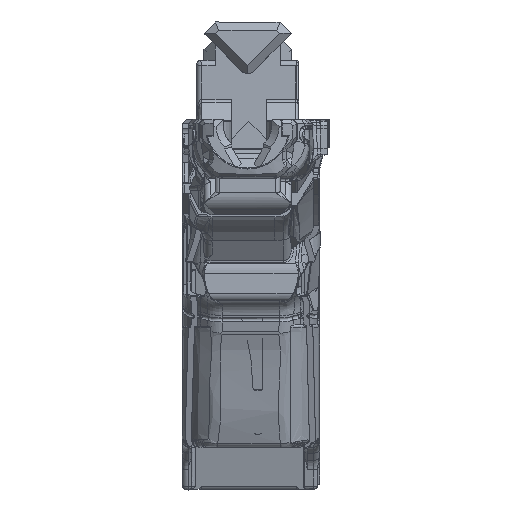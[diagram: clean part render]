
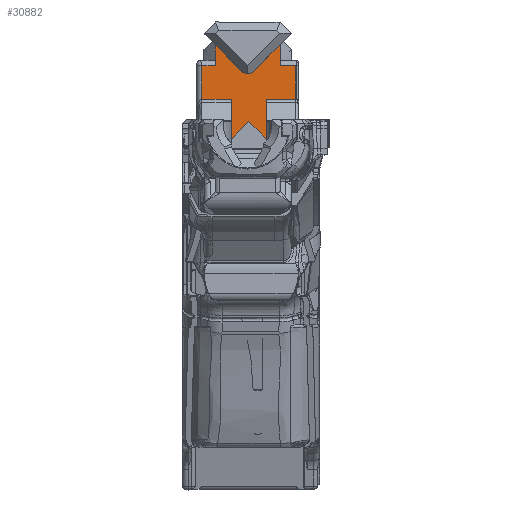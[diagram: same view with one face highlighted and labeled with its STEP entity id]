
A CAD part, left-side view. The second image highlights one B-rep face of the part: STEP entity #30882.
In plain terms, the highlighted planar face has unit normal (-1, 0, 0).
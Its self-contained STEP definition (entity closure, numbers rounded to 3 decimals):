
#1046=PLANE('',#33076);
#3936=FACE_OUTER_BOUND('',#5757,.T.);
#5757=EDGE_LOOP('',(#24518,#24519,#24520,#24521,#24522,#24523,#24524,#24525,
#24526,#24527,#24528,#24529,#24530,#24531,#24532,#24533,#24534));
#7260=CIRCLE('',#33077,2.);
#8450=LINE('',#72859,#10522);
#8471=LINE('',#73172,#10543);
#8473=LINE('',#73192,#10545);
#8594=LINE('',#73938,#10666);
#8595=LINE('',#73940,#10667);
#8596=LINE('',#73942,#10668);
#8597=LINE('',#73944,#10669);
#8598=LINE('',#73946,#10670);
#8599=LINE('',#73948,#10671);
#8600=LINE('',#73949,#10672);
#8601=LINE('',#73951,#10673);
#8602=LINE('',#73953,#10674);
#8603=LINE('',#73955,#10675);
#8604=LINE('',#73959,#10676);
#8605=LINE('',#73961,#10677);
#8606=LINE('',#73962,#10678);
#10522=VECTOR('',#37167,1000.);
#10543=VECTOR('',#37262,1000.);
#10545=VECTOR('',#37270,1000.);
#10666=VECTOR('',#37631,1000.);
#10667=VECTOR('',#37632,1000.);
#10668=VECTOR('',#37633,1000.);
#10669=VECTOR('',#37634,1000.);
#10670=VECTOR('',#37635,1000.);
#10671=VECTOR('',#37636,1000.);
#10672=VECTOR('',#37637,1000.);
#10673=VECTOR('',#37638,1000.);
#10674=VECTOR('',#37639,1000.);
#10675=VECTOR('',#37640,1000.);
#10676=VECTOR('',#37643,1000.);
#10677=VECTOR('',#37644,1000.);
#10678=VECTOR('',#37645,1000.);
#13670=VERTEX_POINT('',#72698);
#13673=VERTEX_POINT('',#72779);
#13728=VERTEX_POINT('',#73168);
#13730=VERTEX_POINT('',#73171);
#13735=VERTEX_POINT('',#73191);
#13919=VERTEX_POINT('',#73937);
#13920=VERTEX_POINT('',#73939);
#13921=VERTEX_POINT('',#73941);
#13922=VERTEX_POINT('',#73943);
#13923=VERTEX_POINT('',#73945);
#13924=VERTEX_POINT('',#73947);
#13925=VERTEX_POINT('',#73950);
#13926=VERTEX_POINT('',#73952);
#13927=VERTEX_POINT('',#73954);
#13928=VERTEX_POINT('',#73956);
#13929=VERTEX_POINT('',#73958);
#13930=VERTEX_POINT('',#73960);
#17495=EDGE_CURVE('',#13673,#13670,#8450,.T.);
#17561=EDGE_CURVE('',#13728,#13730,#8471,.T.);
#17567=EDGE_CURVE('',#13670,#13735,#8473,.T.);
#17792=EDGE_CURVE('',#13673,#13919,#8594,.T.);
#17793=EDGE_CURVE('',#13919,#13920,#8595,.T.);
#17794=EDGE_CURVE('',#13920,#13921,#8596,.T.);
#17795=EDGE_CURVE('',#13921,#13922,#8597,.T.);
#17796=EDGE_CURVE('',#13923,#13922,#8598,.T.);
#17797=EDGE_CURVE('',#13923,#13924,#8599,.T.);
#17798=EDGE_CURVE('',#13730,#13924,#8600,.T.);
#17799=EDGE_CURVE('',#13925,#13728,#8601,.T.);
#17800=EDGE_CURVE('',#13926,#13925,#8602,.T.);
#17801=EDGE_CURVE('',#13927,#13926,#8603,.T.);
#17802=EDGE_CURVE('',#13927,#13928,#7260,.T.);
#17803=EDGE_CURVE('',#13928,#13929,#8604,.T.);
#17804=EDGE_CURVE('',#13929,#13930,#8605,.T.);
#17805=EDGE_CURVE('',#13930,#13735,#8606,.T.);
#24518=ORIENTED_EDGE('',*,*,#17495,.F.);
#24519=ORIENTED_EDGE('',*,*,#17792,.T.);
#24520=ORIENTED_EDGE('',*,*,#17793,.T.);
#24521=ORIENTED_EDGE('',*,*,#17794,.T.);
#24522=ORIENTED_EDGE('',*,*,#17795,.T.);
#24523=ORIENTED_EDGE('',*,*,#17796,.F.);
#24524=ORIENTED_EDGE('',*,*,#17797,.T.);
#24525=ORIENTED_EDGE('',*,*,#17798,.F.);
#24526=ORIENTED_EDGE('',*,*,#17561,.F.);
#24527=ORIENTED_EDGE('',*,*,#17799,.F.);
#24528=ORIENTED_EDGE('',*,*,#17800,.F.);
#24529=ORIENTED_EDGE('',*,*,#17801,.F.);
#24530=ORIENTED_EDGE('',*,*,#17802,.T.);
#24531=ORIENTED_EDGE('',*,*,#17803,.T.);
#24532=ORIENTED_EDGE('',*,*,#17804,.T.);
#24533=ORIENTED_EDGE('',*,*,#17805,.T.);
#24534=ORIENTED_EDGE('',*,*,#17567,.F.);
#30882=ADVANCED_FACE('',(#3936),#1046,.T.);
#33076=AXIS2_PLACEMENT_3D('',#73936,#37629,#37630);
#33077=AXIS2_PLACEMENT_3D('',#73957,#37641,#37642);
#37167=DIRECTION('',(0.,0.,1.));
#37262=DIRECTION('',(0.,-1.,0.));
#37270=DIRECTION('',(0.,-1.,0.));
#37629=DIRECTION('center_axis',(-1.,0.,0.));
#37630=DIRECTION('ref_axis',(0.,1.,0.));
#37631=DIRECTION('',(0.,-1.,0.));
#37632=DIRECTION('',(0.,0.,-1.));
#37633=DIRECTION('',(0.,-0.707,0.707));
#37634=DIRECTION('',(0.,-0.707,-0.707));
#37635=DIRECTION('',(0.,0.,-1.));
#37636=DIRECTION('',(0.,-1.,0.));
#37637=DIRECTION('',(0.,0.,-1.));
#37638=DIRECTION('',(0.,0.,-1.));
#37639=DIRECTION('',(0.,-1.,0.));
#37640=DIRECTION('',(0.,-0.707,0.707));
#37641=DIRECTION('center_axis',(1.,0.,0.));
#37642=DIRECTION('ref_axis',(0.,0.,
1.));
#37643=DIRECTION('',(0.,0.707,0.707));
#37644=DIRECTION('',(0.,1.,0.));
#37645=DIRECTION('',(0.,0.,-1.));
#72698=CARTESIAN_POINT('',(72.964,81.274,12.919));
#72779=CARTESIAN_POINT('',(72.964,81.274,4.76));
#72859=CARTESIAN_POINT('',(72.964,81.274,-17.335));
#73168=CARTESIAN_POINT('',(72.964,62.271,12.919));
#73171=CARTESIAN_POINT('',(72.964,58.414,12.919));
#73172=CARTESIAN_POINT('',(72.964,77.891,12.919));
#73191=CARTESIAN_POINT('',(72.964,77.949,12.919));
#73192=CARTESIAN_POINT('',(72.964,77.891,12.919));
#73936=CARTESIAN_POINT('Origin',(72.964,70.114,11.428));
#73937=CARTESIAN_POINT('',(72.964,74.08,4.76));
#73938=CARTESIAN_POINT('',(72.964,70.114,4.76));
#73939=CARTESIAN_POINT('',(72.964,74.08,-4.891));
#73940=CARTESIAN_POINT('',(72.964,74.08,-13.142));
#73941=CARTESIAN_POINT('',(72.964,69.844,-0.654));
#73942=CARTESIAN_POINT('',(72.964,67.882,1.307));
#73943=CARTESIAN_POINT('',(72.964,65.607,-4.891));
#73944=CARTESIAN_POINT('',(72.964,71.805,1.307));
#73945=CARTESIAN_POINT('',(72.964,65.607,4.76));
#73946=CARTESIAN_POINT('',(72.964,65.607,-13.142));
#73947=CARTESIAN_POINT('',(72.964,58.414,4.76));
#73948=CARTESIAN_POINT('',(72.964,70.114,4.76));
#73949=CARTESIAN_POINT('',(72.964,58.414,-17.335));
#73950=CARTESIAN_POINT('',(72.964,62.271,17.979));
#73951=CARTESIAN_POINT('',(72.964,62.271,11.428));
#73952=CARTESIAN_POINT('',(72.964,62.274,17.979));
#73953=CARTESIAN_POINT('',(72.964,70.114,17.979));
#73954=CARTESIAN_POINT('',(72.964,68.695,11.558));
#73955=CARTESIAN_POINT('',(72.964,59.509,20.744));
#73956=CARTESIAN_POINT('',(72.964,71.524,11.558));
#73957=CARTESIAN_POINT('Origin',(72.964,70.109,12.973));
#73958=CARTESIAN_POINT('',(72.964,77.944,17.979));
#73959=CARTESIAN_POINT('',(72.964,70.753,10.788));
#73960=CARTESIAN_POINT('',(72.964,77.949,17.979));
#73961=CARTESIAN_POINT('',(72.964,62.279,17.979));
#73962=CARTESIAN_POINT('',(72.964,77.949,10.174));
